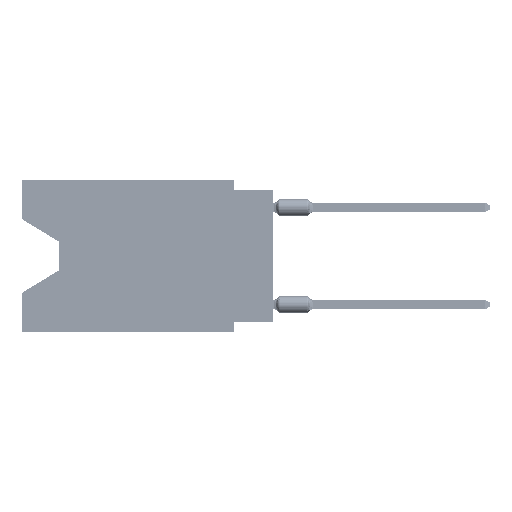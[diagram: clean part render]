
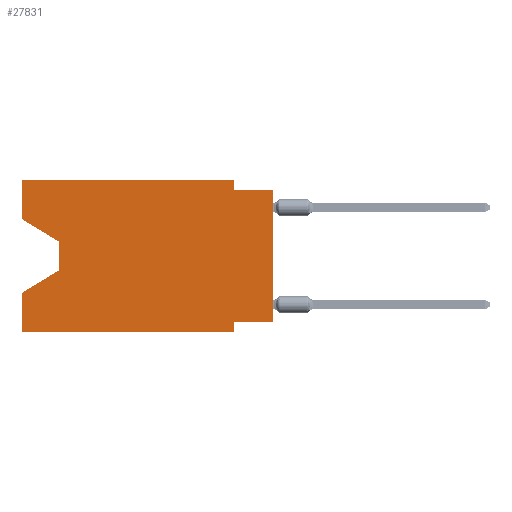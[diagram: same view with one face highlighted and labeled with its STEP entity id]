
A CAD part, left-side view. The second image highlights one B-rep face of the part: STEP entity #27831.
In plain terms, the highlighted planar face has unit normal (-1, 0, 0).
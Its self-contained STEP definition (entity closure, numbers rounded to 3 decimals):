
#345 = LINE ( 'NONE', #12735, #7431 ) ;
#1570 = CARTESIAN_POINT ( 'NONE',  ( 0., 13.97, -4.013 ) ) ;
#2502 = ORIENTED_EDGE ( 'NONE', *, *, #60258, .T. ) ;
#2629 = LINE ( 'NONE', #80806, #12648 ) ;
#4523 = EDGE_CURVE ( 'NONE', #62806, #30804, #345, .T. ) ;
#4531 = VERTEX_POINT ( 'NONE', #18731 ) ;
#5440 = DIRECTION ( 'NONE',  ( 0., 0., 1. ) ) ;
#7044 = VERTEX_POINT ( 'NONE', #31676 ) ;
#7431 = VECTOR ( 'NONE', #19571, 1000. ) ;
#8040 = ORIENTED_EDGE ( 'NONE', *, *, #71554, .T. ) ;
#9021 = DIRECTION ( 'NONE',  ( 0., 0., -1. ) ) ;
#10316 = ORIENTED_EDGE ( 'NONE', *, *, #56110, .F. ) ;
#10448 = DIRECTION ( 'NONE',  ( 0., -1., 0. ) ) ;
#11843 = CARTESIAN_POINT ( 'NONE',  ( 0., 16.383, 0. ) ) ;
#12302 = VERTEX_POINT ( 'NONE', #71275 ) ;
#12452 = FACE_OUTER_BOUND ( 'NONE', #29152, .T. ) ;
#12648 = VECTOR ( 'NONE', #9021, 1000. ) ;
#12735 = CARTESIAN_POINT ( 'NONE',  ( 0., 16.383, 0. ) ) ;
#13205 = CARTESIAN_POINT ( 'NONE',  ( 0., 2.54, 0. ) ) ;
#14537 = VERTEX_POINT ( 'NONE', #60810 ) ;
#14799 = CARTESIAN_POINT ( 'NONE',  ( 0., 0., 0. ) ) ;
#17424 = CARTESIAN_POINT ( 'NONE',  ( 0., 13.97, -5.893 ) ) ;
#17471 = VECTOR ( 'NONE', #70663, 1000. ) ;
#17609 = CARTESIAN_POINT ( 'NONE',  ( 0., 16.383, -2.546 ) ) ;
#18149 = CARTESIAN_POINT ( 'NONE',  ( 0., 2.54, -9.271 ) ) ;
#18229 = CARTESIAN_POINT ( 'NONE',  ( 0., 2.54, 0. ) ) ;
#18573 = CARTESIAN_POINT ( 'NONE',  ( 0., 16.383, -9.906 ) ) ;
#18731 = CARTESIAN_POINT ( 'NONE',  ( 0., 0., -0.635 ) ) ;
#19045 = AXIS2_PLACEMENT_3D ( 'NONE', #65010, #71836, #51777 ) ;
#19571 = DIRECTION ( 'NONE',  ( 0., 0., 1. ) ) ;
#21837 = CARTESIAN_POINT ( 'NONE',  ( 0., 16.383, 0. ) ) ;
#22111 = LINE ( 'NONE', #65713, #39230 ) ;
#24302 = CARTESIAN_POINT ( 'NONE',  ( 0., 0., -9.271 ) ) ;
#25789 = CARTESIAN_POINT ( 'NONE',  ( 0., 13.97, -4.013 ) ) ;
#26056 = VERTEX_POINT ( 'NONE', #24302 ) ;
#27831 = ADVANCED_FACE ( 'NONE', ( #12452 ), #59021, .F. ) ;
#27949 = VERTEX_POINT ( 'NONE', #21837 ) ;
#28189 = ORIENTED_EDGE ( 'NONE', *, *, #83623, .T. ) ;
#29152 = EDGE_LOOP ( 'NONE', ( #66185, #28189, #8040, #37240, #78412, #53400, #37943, #2502, #10316, #33541, #53580, #63819 ) ) ;
#29389 = DIRECTION ( 'NONE',  ( 0., 0.855, -0.519 ) ) ;
#30512 = CARTESIAN_POINT ( 'NONE',  ( 0., 16.383, 0. ) ) ;
#30804 = VERTEX_POINT ( 'NONE', #59048 ) ;
#31485 = DIRECTION ( 'NONE',  ( 0., -1., 0. ) ) ;
#31676 = CARTESIAN_POINT ( 'NONE',  ( 0., 2.54, -9.906 ) ) ;
#32305 = VERTEX_POINT ( 'NONE', #13205 ) ;
#33541 = ORIENTED_EDGE ( 'NONE', *, *, #80619, .F. ) ;
#33737 = CARTESIAN_POINT ( 'NONE',  ( 0., 16.383, -9.906 ) ) ;
#34445 = DIRECTION ( 'NONE',  ( 0., 0., 1. ) ) ;
#35914 = VECTOR ( 'NONE', #31485, 1000. ) ;
#37025 = EDGE_CURVE ( 'NONE', #62806, #7044, #83114, .T. ) ;
#37240 = ORIENTED_EDGE ( 'NONE', *, *, #4523, .F. ) ;
#37341 = LINE ( 'NONE', #25789, #17471 ) ;
#37943 = ORIENTED_EDGE ( 'NONE', *, *, #83050, .F. ) ;
#38738 = CARTESIAN_POINT ( 'NONE',  ( 0., 0., -0.635 ) ) ;
#39230 = VECTOR ( 'NONE', #69084, 1000. ) ;
#44079 = DIRECTION ( 'NONE',  ( 0., -0.855, -0.519 ) ) ;
#44261 = EDGE_CURVE ( 'NONE', #72105, #7044, #2629, .T. ) ;
#44724 = LINE ( 'NONE', #18229, #50169 ) ;
#45173 = VECTOR ( 'NONE', #29389, 1000. ) ;
#49355 = EDGE_CURVE ( 'NONE', #71667, #70095, #70556, .T. ) ;
#50169 = VECTOR ( 'NONE', #70786, 1000. ) ;
#50931 = VECTOR ( 'NONE', #5440, 1000. ) ;
#51777 = DIRECTION ( 'NONE',  ( 0., 0., -1. ) ) ;
#52734 = VECTOR ( 'NONE', #10448, 1000. ) ;
#53400 = ORIENTED_EDGE ( 'NONE', *, *, #44261, .F. ) ;
#53580 = ORIENTED_EDGE ( 'NONE', *, *, #79839, .F. ) ;
#56110 = EDGE_CURVE ( 'NONE', #14537, #4531, #84464, .T. ) ;
#56212 = EDGE_CURVE ( 'NONE', #71667, #27949, #70374, .T. ) ;
#59021 = PLANE ( 'NONE',  #19045 ) ;
#59048 = CARTESIAN_POINT ( 'NONE',  ( 0., 16.383, -7.36 ) ) ;
#60258 = EDGE_CURVE ( 'NONE', #26056, #4531, #61372, .T. ) ;
#60810 = CARTESIAN_POINT ( 'NONE',  ( 0., 2.54, -0.635 ) ) ;
#61372 = LINE ( 'NONE', #14799, #70432 ) ;
#62300 = LINE ( 'NONE', #17424, #45173 ) ;
#62806 = VERTEX_POINT ( 'NONE', #33737 ) ;
#63819 = ORIENTED_EDGE ( 'NONE', *, *, #56212, .F. ) ;
#65010 = CARTESIAN_POINT ( 'NONE',  ( 0., 16.383, 0. ) ) ;
#65236 = CARTESIAN_POINT ( 'NONE',  ( 0., 16.383, -2.546 ) ) ;
#65713 = CARTESIAN_POINT ( 'NONE',  ( 0., 0., -9.271 ) ) ;
#66185 = ORIENTED_EDGE ( 'NONE', *, *, #49355, .T. ) ;
#69084 = DIRECTION ( 'NONE',  ( 0., 1., 0. ) ) ;
#69169 = VECTOR ( 'NONE', #69873, 1000. ) ;
#69873 = DIRECTION ( 'NONE',  ( 0., -1., 0. ) ) ;
#70095 = VERTEX_POINT ( 'NONE', #1570 ) ;
#70374 = LINE ( 'NONE', #11843, #50931 ) ;
#70432 = VECTOR ( 'NONE', #34445, 1000. ) ;
#70556 = LINE ( 'NONE', #17609, #84037 ) ;
#70663 = DIRECTION ( 'NONE',  ( 0., 0., -1. ) ) ;
#70786 = DIRECTION ( 'NONE',  ( 0., 0., -1. ) ) ;
#71275 = CARTESIAN_POINT ( 'NONE',  ( 0., 13.97, -5.893 ) ) ;
#71554 = EDGE_CURVE ( 'NONE', #12302, #30804, #62300, .T. ) ;
#71667 = VERTEX_POINT ( 'NONE', #65236 ) ;
#71836 = DIRECTION ( 'NONE',  ( 1., 0., 0. ) ) ;
#72105 = VERTEX_POINT ( 'NONE', #18149 ) ;
#78412 = ORIENTED_EDGE ( 'NONE', *, *, #37025, .T. ) ;
#79839 = EDGE_CURVE ( 'NONE', #27949, #32305, #83471, .T. ) ;
#80619 = EDGE_CURVE ( 'NONE', #32305, #14537, #44724, .T. ) ;
#80806 = CARTESIAN_POINT ( 'NONE',  ( 0., 2.54, -9.906 ) ) ;
#83050 = EDGE_CURVE ( 'NONE', #26056, #72105, #22111, .T. ) ;
#83114 = LINE ( 'NONE', #18573, #69169 ) ;
#83471 = LINE ( 'NONE', #30512, #52734 ) ;
#83623 = EDGE_CURVE ( 'NONE', #70095, #12302, #37341, .T. ) ;
#84037 = VECTOR ( 'NONE', #44079, 1000. ) ;
#84464 = LINE ( 'NONE', #38738, #35914 ) ;
